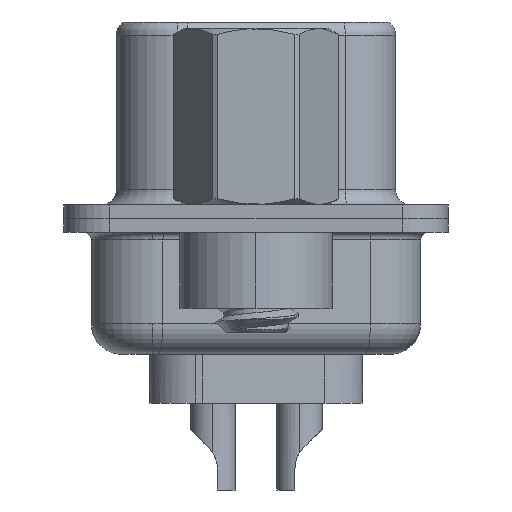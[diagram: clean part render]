
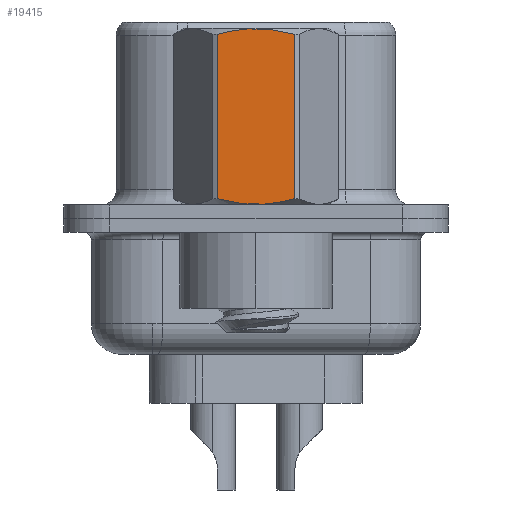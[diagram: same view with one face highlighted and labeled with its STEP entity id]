
A CAD part, left-side view. The second image highlights one B-rep face of the part: STEP entity #19415.
In plain terms, the highlighted planar face has unit normal (-1, 0, 0).
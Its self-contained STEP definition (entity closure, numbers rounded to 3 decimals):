
#1063 = FACE_OUTER_BOUND ( 'NONE', #13172, .T. ) ;
#1617 = ORIENTED_EDGE ( 'NONE', *, *, #14672, .T. ) ;
#1757 = B_SPLINE_CURVE_WITH_KNOTS ( 'NONE', 3,
 ( #18921, #15774, #12274, #7512, #2850, #20402, #18708, #7834, #13972, #6123 ),
 .UNSPECIFIED., .F., .F.,
 ( 4, 2, 2, 2, 4 ),
 ( 0.001, 0.002, 0.002, 0.003, 0.004 ),
 .UNSPECIFIED. ) ;
#2009 = EDGE_CURVE ( 'NONE', #3460, #14886, #9155, .T. ) ;
#2850 = CARTESIAN_POINT ( 'NONE',  ( -2.381, -0.215, 6.232 ) ) ;
#3089 = CARTESIAN_POINT ( 'NONE',  ( -2.381, -1.273, 6.048 ) ) ;
#3460 = VERTEX_POINT ( 'NONE', #20037 ) ;
#5551 = ORIENTED_EDGE ( 'NONE', *, *, #2009, .T. ) ;
#5748 = CARTESIAN_POINT ( 'NONE',  ( -2.381, 0.853, 0.549 ) ) ;
#5778 = VERTEX_POINT ( 'NONE', #3089 ) ;
#5794 = CARTESIAN_POINT ( 'NONE',  ( -2.381, -1.273, 3.792 ) ) ;
#5863 = CARTESIAN_POINT ( 'NONE',  ( -2.381, -0.858, 0.55 ) ) ;
#5928 = PLANE ( 'NONE',  #16980 ) ;
#6123 = CARTESIAN_POINT ( 'NONE',  ( -2.381, 1.273, 6.048 ) ) ;
#6245 = CARTESIAN_POINT ( 'NONE',  ( -2.381, 1.375, -3.75 ) ) ;
#6282 = CARTESIAN_POINT ( 'NONE',  ( -2.381, -1.273, 0.652 ) ) ;
#6511 = CARTESIAN_POINT ( 'NONE',  ( -2.381, 1.273, 0.652 ) ) ;
#7230 = EDGE_CURVE ( 'NONE', #5778, #3460, #1757, .T. ) ;
#7512 = CARTESIAN_POINT ( 'NONE',  ( -2.381, -0.432, 6.215 ) ) ;
#7780 = CARTESIAN_POINT ( 'NONE',  ( -2.381, 1.273, 0.652 ) ) ;
#7834 = CARTESIAN_POINT ( 'NONE',  ( -2.381, 0.853, 6.151 ) ) ;
#8759 = EDGE_CURVE ( 'NONE', #14886, #16862, #19771, .T. ) ;
#8897 = LINE ( 'NONE', #5794, #18562 ) ;
#8988 = ORIENTED_EDGE ( 'NONE', *, *, #7230, .T. ) ;
#9050 = CARTESIAN_POINT ( 'NONE',  ( -2.381, 1.273, 3.792 ) ) ;
#9155 = LINE ( 'NONE', #9050, #12555 ) ;
#12274 = CARTESIAN_POINT ( 'NONE',  ( -2.381, -0.858, 6.15 ) ) ;
#12331 = CARTESIAN_POINT ( 'NONE',  ( -2.381, -1.066, 0.596 ) ) ;
#12555 = VECTOR ( 'NONE', #13690, 1000. ) ;
#12704 = DIRECTION ( 'NONE',  ( -1., 0., 0. ) ) ;
#13172 = EDGE_LOOP ( 'NONE', ( #19264, #1617, #8988, #5551 ) ) ;
#13442 = DIRECTION ( 'NONE',  ( 0., 0., 1. ) ) ;
#13690 = DIRECTION ( 'NONE',  ( 0., 0., -1. ) ) ;
#13972 = CARTESIAN_POINT ( 'NONE',  ( -2.381, 1.065, 6.104 ) ) ;
#14231 = CARTESIAN_POINT ( 'NONE',  ( -2.381, 0.428, 0.485 ) ) ;
#14397 = DIRECTION ( 'NONE',  ( 0., -1., 0. ) ) ;
#14672 = EDGE_CURVE ( 'NONE', #16862, #5778, #8897, .T. ) ;
#14886 = VERTEX_POINT ( 'NONE', #6511 ) ;
#15774 = CARTESIAN_POINT ( 'NONE',  ( -2.381, -1.066, 6.104 ) ) ;
#16862 = VERTEX_POINT ( 'NONE', #6282 ) ;
#16980 = AXIS2_PLACEMENT_3D ( 'NONE', #6245, #12704, #14397 ) ;
#18562 = VECTOR ( 'NONE', #13442, 1000. ) ;
#18708 = CARTESIAN_POINT ( 'NONE',  ( -2.381, 0.428, 6.215 ) ) ;
#18768 = CARTESIAN_POINT ( 'NONE',  ( -2.381, -1.273, 0.652 ) ) ;
#18921 = CARTESIAN_POINT ( 'NONE',  ( -2.381, -1.273, 6.048 ) ) ;
#19264 = ORIENTED_EDGE ( 'NONE', *, *, #8759, .T. ) ;
#19415 = ADVANCED_FACE ( 'NONE', ( #1063 ), #5928, .T. ) ;
#19771 = B_SPLINE_CURVE_WITH_KNOTS ( 'NONE', 3,
 ( #7780, #20565, #5748, #14231, #20355, #20247, #20675, #5863, #12331, #18768 ),
 .UNSPECIFIED., .F., .F.,
 ( 4, 2, 2, 2, 4 ),
 ( 0.003, 0.003, 0.004, 0.004, 0.005 ),
 .UNSPECIFIED. ) ;
#20037 = CARTESIAN_POINT ( 'NONE',  ( -2.381, 1.273, 6.048 ) ) ;
#20247 = CARTESIAN_POINT ( 'NONE',  ( -2.381, -0.215, 0.468 ) ) ;
#20355 = CARTESIAN_POINT ( 'NONE',  ( -2.381, 0.215, 0.468 ) ) ;
#20402 = CARTESIAN_POINT ( 'NONE',  ( -2.381, 0.215, 6.232 ) ) ;
#20565 = CARTESIAN_POINT ( 'NONE',  ( -2.381, 1.065, 0.596 ) ) ;
#20675 = CARTESIAN_POINT ( 'NONE',  ( -2.381, -0.432, 0.485 ) ) ;
